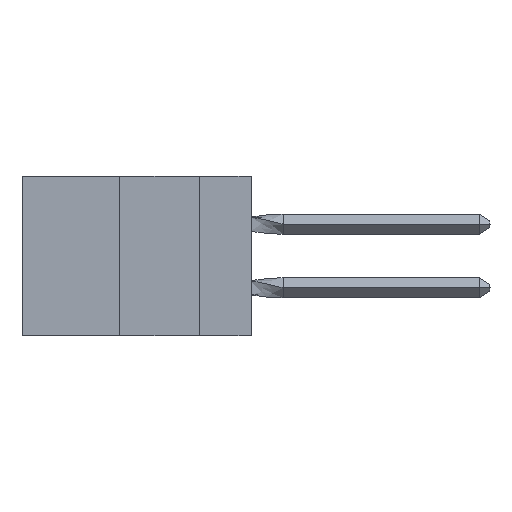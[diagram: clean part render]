
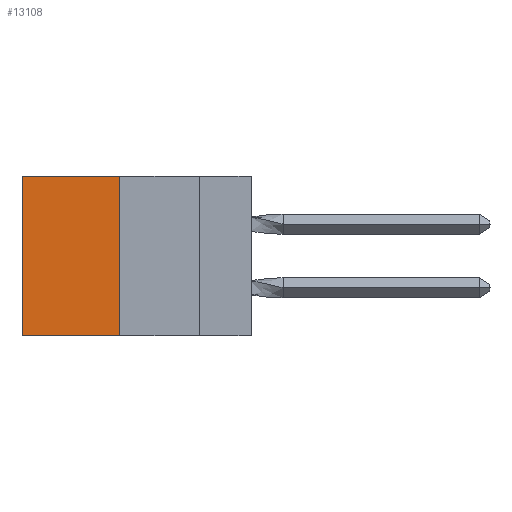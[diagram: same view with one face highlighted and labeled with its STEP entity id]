
A CAD part, left-side view. The second image highlights one B-rep face of the part: STEP entity #13108.
In plain terms, the highlighted planar face has unit normal (-1, 0, 0).
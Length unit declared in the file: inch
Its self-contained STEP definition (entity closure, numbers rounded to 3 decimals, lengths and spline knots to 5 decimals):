
#1111 = PLANE ( 'NONE',  #32947 ) ;
#3256 = ORIENTED_EDGE ( 'NONE', *, *, #27427, .F. ) ;
#3393 = CARTESIAN_POINT ( 'NONE',  ( 0.305, 0.413, -0.5 ) ) ;
#3698 = EDGE_CURVE ( 'NONE', #29648, #19582, #26583, .T. ) ;
#3957 = DIRECTION ( 'NONE',  ( 0., 0., -1. ) ) ;
#4423 = CARTESIAN_POINT ( 'NONE',  ( 0.305, 0.72, -0.5 ) ) ;
#6560 = CARTESIAN_POINT ( 'NONE',  ( 0.305, 0.72, -0.5 ) ) ;
#6808 = CARTESIAN_POINT ( 'NONE',  ( 0.305, 0.413, -0.5 ) ) ;
#6950 = EDGE_CURVE ( 'NONE', #23269, #22189, #12560, .T. ) ;
#7094 = CARTESIAN_POINT ( 'NONE',  ( 0.305, 0.413, -0.5 ) ) ;
#10743 = CARTESIAN_POINT ( 'NONE',  ( 0.305, 0.413, 0. ) ) ;
#11352 = EDGE_LOOP ( 'NONE', ( #21449, #3256, #31873, #16242 ) ) ;
#12560 = LINE ( 'NONE', #23100, #31667 ) ;
#12814 = VECTOR ( 'NONE', #28168, 39.37008 ) ;
#12844 = DIRECTION ( 'NONE',  ( 1., 0., 0. ) ) ;
#13108 = ADVANCED_FACE ( 'NONE', ( #29286 ), #1111, .F. ) ;
#15347 = CARTESIAN_POINT ( 'NONE',  ( 0.305, 0.72, 0. ) ) ;
#16242 = ORIENTED_EDGE ( 'NONE', *, *, #24749, .T. ) ;
#18801 = DIRECTION ( 'NONE',  ( 0., 0., -1. ) ) ;
#19582 = VERTEX_POINT ( 'NONE', #6560 ) ;
#21449 = ORIENTED_EDGE ( 'NONE', *, *, #3698, .T. ) ;
#22189 = VERTEX_POINT ( 'NONE', #3393 ) ;
#23100 = CARTESIAN_POINT ( 'NONE',  ( 0.305, 0.413, -0.5 ) ) ;
#23269 = VERTEX_POINT ( 'NONE', #10743 ) ;
#24749 = EDGE_CURVE ( 'NONE', #23269, #29648, #31674, .T. ) ;
#25661 = VECTOR ( 'NONE', #18801, 39.37008 ) ;
#25917 = CARTESIAN_POINT ( 'NONE',  ( 0.305, 0.413, 0. ) ) ;
#26583 = LINE ( 'NONE', #4423, #25661 ) ;
#27427 = EDGE_CURVE ( 'NONE', #22189, #19582, #32864, .T. ) ;
#28168 = DIRECTION ( 'NONE',  ( 0., 1., 0. ) ) ;
#29117 = DIRECTION ( 'NONE',  ( 0., 0., -1. ) ) ;
#29286 = FACE_OUTER_BOUND ( 'NONE', #11352, .T. ) ;
#29648 = VERTEX_POINT ( 'NONE', #15347 ) ;
#31667 = VECTOR ( 'NONE', #29117, 39.37008 ) ;
#31674 = LINE ( 'NONE', #25917, #36837 ) ;
#31873 = ORIENTED_EDGE ( 'NONE', *, *, #6950, .F. ) ;
#32864 = LINE ( 'NONE', #6808, #12814 ) ;
#32947 = AXIS2_PLACEMENT_3D ( 'NONE', #7094, #12844, #3957 ) ;
#34808 = DIRECTION ( 'NONE',  ( 0., 1., 0. ) ) ;
#36837 = VECTOR ( 'NONE', #34808, 39.37008 ) ;
